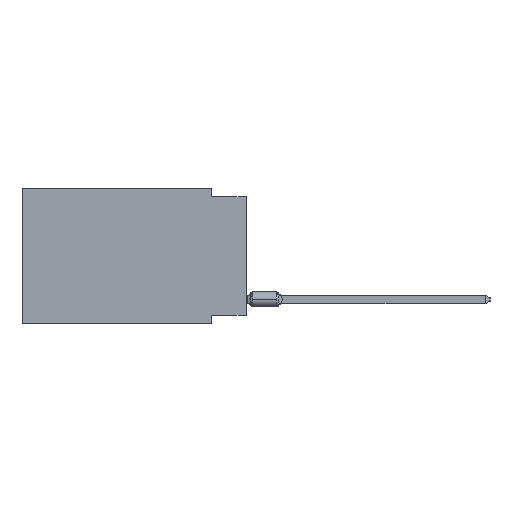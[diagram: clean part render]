
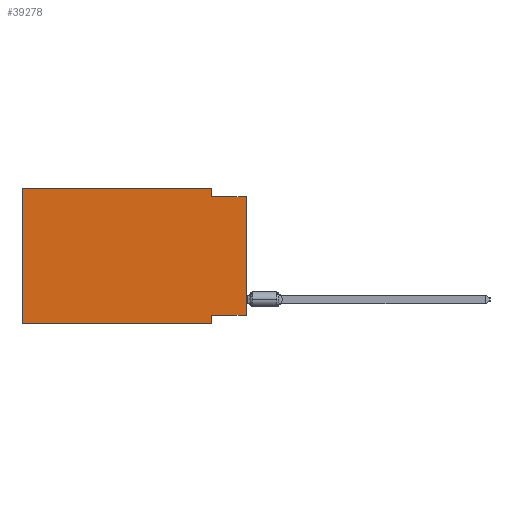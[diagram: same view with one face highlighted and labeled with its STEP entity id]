
A CAD part, left-side view. The second image highlights one B-rep face of the part: STEP entity #39278.
In plain terms, the highlighted planar face has unit normal (-1, 0, 0).
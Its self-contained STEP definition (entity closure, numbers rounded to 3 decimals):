
#744 = EDGE_CURVE ( 'NONE', #41926, #41348, #57773, .T. ) ;
#1477 = EDGE_CURVE ( 'NONE', #41926, #39904, #56813, .T. ) ;
#1950 = VERTEX_POINT ( 'NONE', #57510 ) ;
#2442 = LINE ( 'NONE', #19224, #14846 ) ;
#2966 = CARTESIAN_POINT ( 'NONE',  ( 0., 0., 0. ) ) ;
#4113 = DIRECTION ( 'NONE',  ( 0., 0., -1. ) ) ;
#4334 = EDGE_CURVE ( 'NONE', #18208, #41041, #48692, .T. ) ;
#4806 = ORIENTED_EDGE ( 'NONE', *, *, #4334, .F. ) ;
#7987 = EDGE_LOOP ( 'NONE', ( #9261, #15933, #12103, #4806, #66112, #23096, #43146, #62974 ) ) ;
#9261 = ORIENTED_EDGE ( 'NONE', *, *, #1477, .T. ) ;
#9568 = CARTESIAN_POINT ( 'NONE',  ( 0., 0., -0.635 ) ) ;
#9748 = DIRECTION ( 'NONE',  ( 0., 0., 1. ) ) ;
#10517 = VECTOR ( 'NONE', #26033, 1000. ) ;
#12103 = ORIENTED_EDGE ( 'NONE', *, *, #65961, .F. ) ;
#12883 = CARTESIAN_POINT ( 'NONE',  ( 0., 16.383, 0. ) ) ;
#14350 = EDGE_CURVE ( 'NONE', #1950, #14417, #47407, .T. ) ;
#14417 = VERTEX_POINT ( 'NONE', #33587 ) ;
#14846 = VECTOR ( 'NONE', #20383, 1000. ) ;
#15933 = ORIENTED_EDGE ( 'NONE', *, *, #69719, .F. ) ;
#16779 = CARTESIAN_POINT ( 'NONE',  ( 0., 0., -9.271 ) ) ;
#17131 = LINE ( 'NONE', #22600, #47940 ) ;
#17160 = DIRECTION ( 'NONE',  ( 0., 1., 0. ) ) ;
#18208 = VERTEX_POINT ( 'NONE', #50670 ) ;
#18897 = CARTESIAN_POINT ( 'NONE',  ( 0., 16.383, -9.906 ) ) ;
#19224 = CARTESIAN_POINT ( 'NONE',  ( 0., 0., -0.635 ) ) ;
#20383 = DIRECTION ( 'NONE',  ( 0., -1., 0. ) ) ;
#21349 = VECTOR ( 'NONE', #17160, 1000. ) ;
#21468 = CARTESIAN_POINT ( 'NONE',  ( 0., 2.54, -0.635 ) ) ;
#21584 = DIRECTION ( 'NONE',  ( 0., 0., -1. ) ) ;
#22600 = CARTESIAN_POINT ( 'NONE',  ( 0., 16.383, 0. ) ) ;
#23096 = ORIENTED_EDGE ( 'NONE', *, *, #14350, .T. ) ;
#23967 = DIRECTION ( 'NONE',  ( 0., -1., 0. ) ) ;
#26033 = DIRECTION ( 'NONE',  ( 0., -1., 0. ) ) ;
#28795 = EDGE_CURVE ( 'NONE', #41348, #14417, #33762, .T. ) ;
#29665 = PLANE ( 'NONE',  #34465 ) ;
#33587 = CARTESIAN_POINT ( 'NONE',  ( 0., 2.54, -9.906 ) ) ;
#33762 = LINE ( 'NONE', #57588, #69721 ) ;
#34465 = AXIS2_PLACEMENT_3D ( 'NONE', #12883, #54238, #36668 ) ;
#34527 = CARTESIAN_POINT ( 'NONE',  ( 0., 2.54, 0. ) ) ;
#36668 = DIRECTION ( 'NONE',  ( 0., 0., -1. ) ) ;
#36758 = VECTOR ( 'NONE', #23967, 1000. ) ;
#39278 = ADVANCED_FACE ( 'NONE', ( #71404 ), #29665, .F. ) ;
#39904 = VERTEX_POINT ( 'NONE', #9568 ) ;
#41041 = VERTEX_POINT ( 'NONE', #34527 ) ;
#41348 = VERTEX_POINT ( 'NONE', #68038 ) ;
#41926 = VERTEX_POINT ( 'NONE', #60750 ) ;
#43146 = ORIENTED_EDGE ( 'NONE', *, *, #28795, .F. ) ;
#47407 = LINE ( 'NONE', #18897, #36758 ) ;
#47940 = VECTOR ( 'NONE', #9748, 1000. ) ;
#48692 = LINE ( 'NONE', #68170, #10517 ) ;
#50151 = VECTOR ( 'NONE', #50583, 1000. ) ;
#50583 = DIRECTION ( 'NONE',  ( 0., 0., 1. ) ) ;
#50670 = CARTESIAN_POINT ( 'NONE',  ( 0., 16.383, 0. ) ) ;
#51256 = LINE ( 'NONE', #75040, #56793 ) ;
#54238 = DIRECTION ( 'NONE',  ( 1., 0., 0. ) ) ;
#56793 = VECTOR ( 'NONE', #21584, 1000. ) ;
#56813 = LINE ( 'NONE', #2966, #50151 ) ;
#57510 = CARTESIAN_POINT ( 'NONE',  ( 0., 16.383, -9.906 ) ) ;
#57588 = CARTESIAN_POINT ( 'NONE',  ( 0., 2.54, -9.906 ) ) ;
#57773 = LINE ( 'NONE', #16779, #21349 ) ;
#60750 = CARTESIAN_POINT ( 'NONE',  ( 0., 0., -9.271 ) ) ;
#62974 = ORIENTED_EDGE ( 'NONE', *, *, #744, .F. ) ;
#63583 = EDGE_CURVE ( 'NONE', #1950, #18208, #17131, .T. ) ;
#65961 = EDGE_CURVE ( 'NONE', #41041, #71151, #51256, .T. ) ;
#66112 = ORIENTED_EDGE ( 'NONE', *, *, #63583, .F. ) ;
#68038 = CARTESIAN_POINT ( 'NONE',  ( 0., 2.54, -9.271 ) ) ;
#68170 = CARTESIAN_POINT ( 'NONE',  ( 0., 16.383, 0. ) ) ;
#69719 = EDGE_CURVE ( 'NONE', #71151, #39904, #2442, .T. ) ;
#69721 = VECTOR ( 'NONE', #4113, 1000. ) ;
#71151 = VERTEX_POINT ( 'NONE', #21468 ) ;
#71404 = FACE_OUTER_BOUND ( 'NONE', #7987, .T. ) ;
#75040 = CARTESIAN_POINT ( 'NONE',  ( 0., 2.54, 0. ) ) ;
